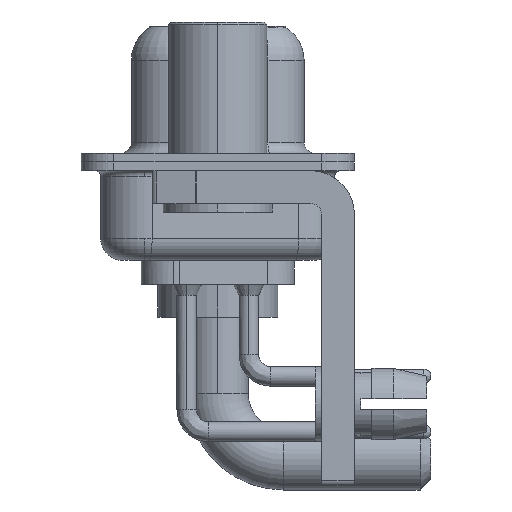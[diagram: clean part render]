
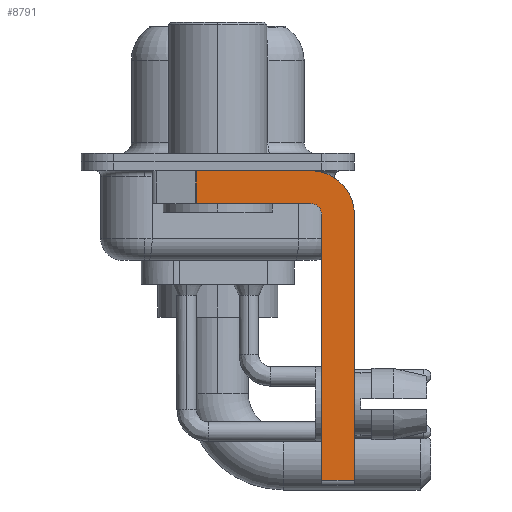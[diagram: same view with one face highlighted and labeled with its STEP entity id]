
A CAD part, left-side view. The second image highlights one B-rep face of the part: STEP entity #8791.
In plain terms, the highlighted planar face has unit normal (-1, 0, 0).
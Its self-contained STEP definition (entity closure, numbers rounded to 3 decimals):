
#24 = CARTESIAN_POINT ( 'NONE',  ( -2.9, 0.978, -1.9 ) ) ;
#70 = DIRECTION ( 'NONE',  ( -1., 0., 0. ) ) ;
#189 = VECTOR ( 'NONE', #7420, 1000. ) ;
#298 = EDGE_CURVE ( 'NONE', #9842, #8928, #21278, .T. ) ;
#565 = CIRCLE ( 'NONE', #3810, 0.5 ) ;
#779 = VERTEX_POINT ( 'NONE', #1003 ) ;
#815 = ORIENTED_EDGE ( 'NONE', *, *, #20882, .T. ) ;
#931 = CARTESIAN_POINT ( 'NONE',  ( -2.9, 3., -0.4 ) ) ;
#1003 = CARTESIAN_POINT ( 'NONE',  ( -2.9, -4.75, -2.4 ) ) ;
#1256 = CARTESIAN_POINT ( 'NONE',  ( -2.9, -4.25, -2.4 ) ) ;
#2044 = CARTESIAN_POINT ( 'NONE',  ( -2.9, 0.978, -1.9 ) ) ;
#2736 = EDGE_LOOP ( 'NONE', ( #19294, #10437, #21626, #20587, #17392, #815, #19356, #4221 ) ) ;
#3487 = DIRECTION ( 'NONE',  ( 0., 0., -1. ) ) ;
#3773 = EDGE_CURVE ( 'NONE', #12954, #21112, #5529, .T. ) ;
#3810 = AXIS2_PLACEMENT_3D ( 'NONE', #5138, #70, #18858 ) ;
#3824 = CARTESIAN_POINT ( 'NONE',  ( -2.9, -4.25, -2.4 ) ) ;
#3853 = DIRECTION ( 'NONE',  ( 0., 0., -1. ) ) ;
#4221 = ORIENTED_EDGE ( 'NONE', *, *, #3773, .F. ) ;
#4420 = LINE ( 'NONE', #931, #13331 ) ;
#4863 = DIRECTION ( 'NONE',  ( 0., 0., 1. ) ) ;
#5138 = CARTESIAN_POINT ( 'NONE',  ( -2.9, -4.25, -2.4 ) ) ;
#5529 = CIRCLE ( 'NONE', #18121, 2. ) ;
#5862 = CARTESIAN_POINT ( 'NONE',  ( -2.9, -4.25, -14.55 ) ) ;
#6065 = VERTEX_POINT ( 'NONE', #16849 ) ;
#6476 = EDGE_CURVE ( 'NONE', #779, #9842, #565, .T. ) ;
#7096 = LINE ( 'NONE', #2044, #13960 ) ;
#7420 = DIRECTION ( 'NONE',  ( 0., 0., -1. ) ) ;
#7678 = VERTEX_POINT ( 'NONE', #14252 ) ;
#8095 = DIRECTION ( 'NONE',  ( 1., 0., 0. ) ) ;
#8199 = AXIS2_PLACEMENT_3D ( 'NONE', #1256, #8095, #9900 ) ;
#8791 = ADVANCED_FACE ( 'NONE', ( #14757 ), #16674, .F. ) ;
#8928 = VERTEX_POINT ( 'NONE', #24 ) ;
#9326 = DIRECTION ( 'NONE',  ( 0., -1., 0. ) ) ;
#9395 = EDGE_CURVE ( 'NONE', #6065, #8928, #7096, .T. ) ;
#9748 = VECTOR ( 'NONE', #9326, 1000. ) ;
#9842 = VERTEX_POINT ( 'NONE', #17323 ) ;
#9900 = DIRECTION ( 'NONE',  ( 0., 0., -1. ) ) ;
#10293 = VECTOR ( 'NONE', #12938, 1000. ) ;
#10437 = ORIENTED_EDGE ( 'NONE', *, *, #9395, .T. ) ;
#10913 = EDGE_CURVE ( 'NONE', #7678, #779, #11267, .T. ) ;
#11083 = VECTOR ( 'NONE', #4863, 1000. ) ;
#11267 = LINE ( 'NONE', #16670, #11083 ) ;
#12518 = CARTESIAN_POINT ( 'NONE',  ( -2.9, -6.25, -14.55 ) ) ;
#12938 = DIRECTION ( 'NONE',  ( 0., 1., 0. ) ) ;
#12954 = VERTEX_POINT ( 'NONE', #18090 ) ;
#13331 = VECTOR ( 'NONE', #16665, 1000. ) ;
#13960 = VECTOR ( 'NONE', #3853, 1000. ) ;
#14082 = CARTESIAN_POINT ( 'NONE',  ( -2.9, -6.25, -2.4 ) ) ;
#14252 = CARTESIAN_POINT ( 'NONE',  ( -2.9, -4.75, -14.55 ) ) ;
#14757 = FACE_OUTER_BOUND ( 'NONE', #2736, .T. ) ;
#15165 = EDGE_CURVE ( 'NONE', #6065, #12954, #4420, .T. ) ;
#15992 = LINE ( 'NONE', #14082, #189 ) ;
#16665 = DIRECTION ( 'NONE',  ( 0., -1., 0. ) ) ;
#16670 = CARTESIAN_POINT ( 'NONE',  ( -2.9, -4.75, -14.8 ) ) ;
#16674 = PLANE ( 'NONE',  #8199 ) ;
#16849 = CARTESIAN_POINT ( 'NONE',  ( -2.9, 0.978, -0.4 ) ) ;
#17323 = CARTESIAN_POINT ( 'NONE',  ( -2.9, -4.25, -1.9 ) ) ;
#17392 = ORIENTED_EDGE ( 'NONE', *, *, #10913, .F. ) ;
#18090 = CARTESIAN_POINT ( 'NONE',  ( -2.9, -4.25, -0.4 ) ) ;
#18095 = VERTEX_POINT ( 'NONE', #12518 ) ;
#18121 = AXIS2_PLACEMENT_3D ( 'NONE', #3824, #18892, #3487 ) ;
#18616 = EDGE_CURVE ( 'NONE', #21112, #18095, #15992, .T. ) ;
#18858 = DIRECTION ( 'NONE',  ( 0., 0., 1. ) ) ;
#18892 = DIRECTION ( 'NONE',  ( 1., 0., 0. ) ) ;
#19294 = ORIENTED_EDGE ( 'NONE', *, *, #15165, .F. ) ;
#19356 = ORIENTED_EDGE ( 'NONE', *, *, #18616, .F. ) ;
#19613 = CARTESIAN_POINT ( 'NONE',  ( -2.9, -6.25, -2.4 ) ) ;
#20587 = ORIENTED_EDGE ( 'NONE', *, *, #6476, .F. ) ;
#20882 = EDGE_CURVE ( 'NONE', #7678, #18095, #21264, .T. ) ;
#21112 = VERTEX_POINT ( 'NONE', #19613 ) ;
#21264 = LINE ( 'NONE', #5862, #9748 ) ;
#21278 = LINE ( 'NONE', #21394, #10293 ) ;
#21394 = CARTESIAN_POINT ( 'NONE',  ( -2.9, -4.25, -1.9 ) ) ;
#21626 = ORIENTED_EDGE ( 'NONE', *, *, #298, .F. ) ;
